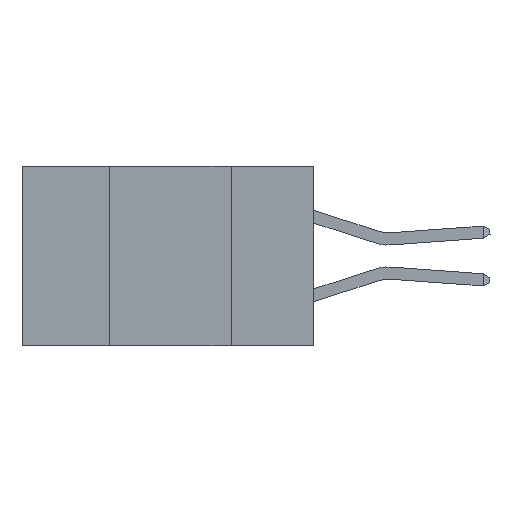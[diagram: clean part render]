
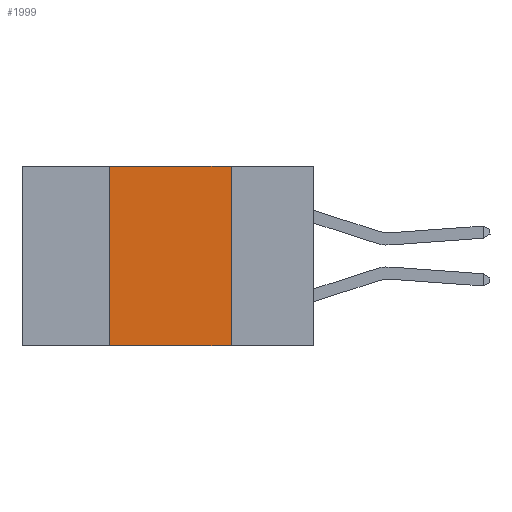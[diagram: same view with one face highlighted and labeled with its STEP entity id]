
A CAD part, left-side view. The second image highlights one B-rep face of the part: STEP entity #1999.
In plain terms, the highlighted planar face has unit normal (-1, 0, 0).
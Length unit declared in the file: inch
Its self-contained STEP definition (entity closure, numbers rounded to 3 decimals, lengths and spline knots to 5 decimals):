
#412 = EDGE_CURVE ( 'NONE', #7997, #1672, #2052, .T. ) ;
#645 = DIRECTION ( 'NONE',  ( 0., -1., 0. ) ) ;
#1113 = VECTOR ( 'NONE', #1412, 39.37008 ) ;
#1226 = VECTOR ( 'NONE', #6469, 39.37008 ) ;
#1230 = PLANE ( 'NONE',  #7884 ) ;
#1232 = LINE ( 'NONE', #5675, #1113 ) ;
#1327 = LINE ( 'NONE', #8722, #5803 ) ;
#1412 = DIRECTION ( 'NONE',  ( 0., 0., -1. ) ) ;
#1672 = VERTEX_POINT ( 'NONE', #3640 ) ;
#1782 = ORIENTED_EDGE ( 'NONE', *, *, #412, .F. ) ;
#1843 = VERTEX_POINT ( 'NONE', #2524 ) ;
#1999 = ADVANCED_FACE ( 'NONE', ( #7258 ), #1230, .F. ) ;
#2052 = LINE ( 'NONE', #3548, #1226 ) ;
#2524 = CARTESIAN_POINT ( 'NONE',  ( 0., 0.42, -0.37 ) ) ;
#2667 = DIRECTION ( 'NONE',  ( 1., 0., 0. ) ) ;
#2797 = CARTESIAN_POINT ( 'NONE',  ( 0., 0.6, 0. ) ) ;
#3201 = EDGE_CURVE ( 'NONE', #1672, #6778, #1232, .T. ) ;
#3544 = ORIENTED_EDGE ( 'NONE', *, *, #5928, .F. ) ;
#3548 = CARTESIAN_POINT ( 'NONE',  ( 0., 0.6, 0. ) ) ;
#3582 = DIRECTION ( 'NONE',  ( 0., 0., -1. ) ) ;
#3640 = CARTESIAN_POINT ( 'NONE',  ( 0., 0.17, 0. ) ) ;
#4836 = VECTOR ( 'NONE', #7074, 39.37008 ) ;
#5367 = EDGE_LOOP ( 'NONE', ( #8831, #1782, #3544, #8869 ) ) ;
#5675 = CARTESIAN_POINT ( 'NONE',  ( 0., 0.17, 0. ) ) ;
#5803 = VECTOR ( 'NONE', #645, 39.37008 ) ;
#5928 = EDGE_CURVE ( 'NONE', #1843, #7997, #9437, .T. ) ;
#6355 = CARTESIAN_POINT ( 'NONE',  ( 0., 0.42, 0. ) ) ;
#6469 = DIRECTION ( 'NONE',  ( 0., -1., 0. ) ) ;
#6778 = VERTEX_POINT ( 'NONE', #7721 ) ;
#7074 = DIRECTION ( 'NONE',  ( 0., 0., 1. ) ) ;
#7258 = FACE_OUTER_BOUND ( 'NONE', #5367, .T. ) ;
#7721 = CARTESIAN_POINT ( 'NONE',  ( 0., 0.17, -0.37 ) ) ;
#7773 = CARTESIAN_POINT ( 'NONE',  ( 0., 0.42, 0. ) ) ;
#7884 = AXIS2_PLACEMENT_3D ( 'NONE', #2797, #2667, #3582 ) ;
#7997 = VERTEX_POINT ( 'NONE', #7773 ) ;
#8690 = EDGE_CURVE ( 'NONE', #1843, #6778, #1327, .T. ) ;
#8722 = CARTESIAN_POINT ( 'NONE',  ( 0., 0.6, -0.37 ) ) ;
#8831 = ORIENTED_EDGE ( 'NONE', *, *, #3201, .F. ) ;
#8869 = ORIENTED_EDGE ( 'NONE', *, *, #8690, .T. ) ;
#9437 = LINE ( 'NONE', #6355, #4836 ) ;
